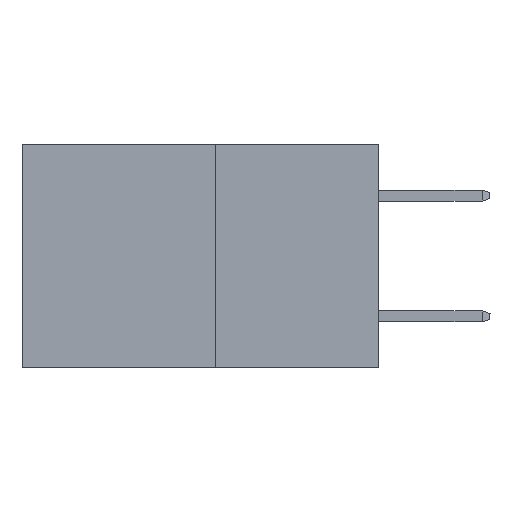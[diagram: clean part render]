
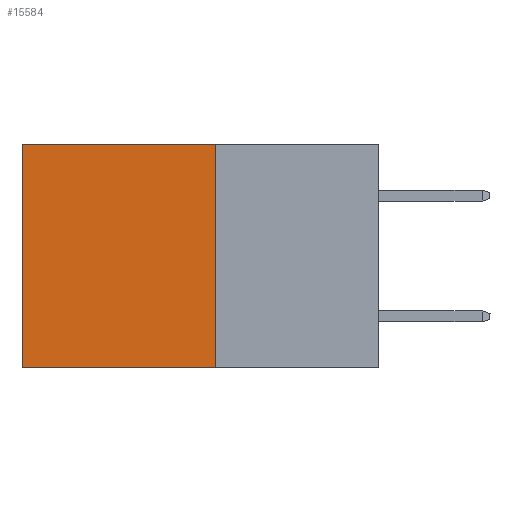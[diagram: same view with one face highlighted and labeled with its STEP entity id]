
A CAD part, left-side view. The second image highlights one B-rep face of the part: STEP entity #15584.
In plain terms, the highlighted planar face has unit normal (-1, 0, 0).
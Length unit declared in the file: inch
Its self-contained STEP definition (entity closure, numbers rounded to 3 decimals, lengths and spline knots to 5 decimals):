
#284 = LINE ( 'NONE', #19431, #28033 ) ;
#1349 = VECTOR ( 'NONE', #27490, 39.37008 ) ;
#2252 = EDGE_CURVE ( 'NONE', #6448, #25897, #284, .T. ) ;
#2291 = EDGE_CURVE ( 'NONE', #6448, #27785, #12976, .T. ) ;
#3428 = CARTESIAN_POINT ( 'NONE',  ( 0.277, 0.59, -0.37 ) ) ;
#5797 = VECTOR ( 'NONE', #16167, 39.37008 ) ;
#6088 = EDGE_LOOP ( 'NONE', ( #24665, #12574, #12600, #23904 ) ) ;
#6448 = VERTEX_POINT ( 'NONE', #13156 ) ;
#7176 = CARTESIAN_POINT ( 'NONE',  ( 0.277, 0.27, -0.37 ) ) ;
#7726 = LINE ( 'NONE', #3428, #1349 ) ;
#8473 = VERTEX_POINT ( 'NONE', #21260 ) ;
#10758 = AXIS2_PLACEMENT_3D ( 'NONE', #33867, #31327, #15340 ) ;
#10921 = CARTESIAN_POINT ( 'NONE',  ( 0.277, 0.27, -0.37 ) ) ;
#11390 = EDGE_CURVE ( 'NONE', #27785, #8473, #24267, .T. ) ;
#12574 = ORIENTED_EDGE ( 'NONE', *, *, #11390, .F. ) ;
#12600 = ORIENTED_EDGE ( 'NONE', *, *, #2291, .F. ) ;
#12719 = DIRECTION ( 'NONE',  ( 0., 1., 0. ) ) ;
#12976 = LINE ( 'NONE', #10921, #5797 ) ;
#13156 = CARTESIAN_POINT ( 'NONE',  ( 0.277, 0.27, 0. ) ) ;
#15340 = DIRECTION ( 'NONE',  ( 0., 0., -1. ) ) ;
#15584 = ADVANCED_FACE ( 'NONE', ( #22542 ), #25983, .F. ) ;
#16167 = DIRECTION ( 'NONE',  ( 0., 0., -1. ) ) ;
#19431 = CARTESIAN_POINT ( 'NONE',  ( 0.277, 0.27, 0. ) ) ;
#20970 = CARTESIAN_POINT ( 'NONE',  ( 0.277, 0.59, 0. ) ) ;
#21260 = CARTESIAN_POINT ( 'NONE',  ( 0.277, 0.59, -0.37 ) ) ;
#22453 = DIRECTION ( 'NONE',  ( 0., 1., 0. ) ) ;
#22542 = FACE_OUTER_BOUND ( 'NONE', #6088, .T. ) ;
#23427 = VECTOR ( 'NONE', #12719, 39.37008 ) ;
#23904 = ORIENTED_EDGE ( 'NONE', *, *, #2252, .T. ) ;
#24267 = LINE ( 'NONE', #7176, #23427 ) ;
#24665 = ORIENTED_EDGE ( 'NONE', *, *, #32478, .T. ) ;
#25897 = VERTEX_POINT ( 'NONE', #20970 ) ;
#25983 = PLANE ( 'NONE',  #10758 ) ;
#26113 = CARTESIAN_POINT ( 'NONE',  ( 0.277, 0.27, -0.37 ) ) ;
#27490 = DIRECTION ( 'NONE',  ( 0., 0., -1. ) ) ;
#27785 = VERTEX_POINT ( 'NONE', #26113 ) ;
#28033 = VECTOR ( 'NONE', #22453, 39.37008 ) ;
#31327 = DIRECTION ( 'NONE',  ( 1., 0., 0. ) ) ;
#32478 = EDGE_CURVE ( 'NONE', #25897, #8473, #7726, .T. ) ;
#33867 = CARTESIAN_POINT ( 'NONE',  ( 0.277, 0.27, -0.37 ) ) ;
